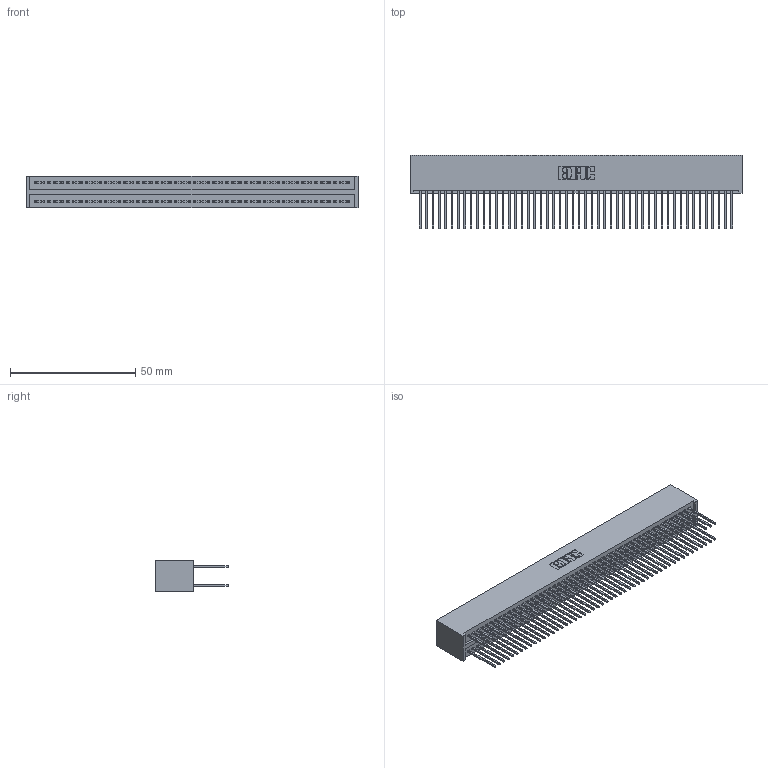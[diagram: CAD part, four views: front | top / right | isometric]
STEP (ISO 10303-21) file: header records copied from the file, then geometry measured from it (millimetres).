
FILE_DESCRIPTION (( 'STEP AP203' ), '1' );
FILE_NAME ('325-100-540-201.STEP', '2020-02-25T06:40:36', ( '' ), ( '' ), 'SwSTEP 2.0', 'SolidWorks 2016', '' );
FILE_SCHEMA (( 'CONFIG_CONTROL_DESIGN' ));
Length unit declared in the file: inch
Products named in the file (3): 325-100-540-201; 325-292-001_325-293-140; 325 Part_Lugless
Assembly tree (101 placements, depth 2):
  325-100-540-201
    325 Part_Lugless
    325-292-001_325-293-140  x100
Bounding box: 132.64 x 29.46 x 12.45 mm (x, y, z)
Volume: 18180.4 mm3; surface area: 24660.2 mm2
Topology: 101 solids, 101 shells, 5306 faces, 15787 edges, 10390 vertices
Faces by surface type: plane 3666, cylinder 1640
Entity records: 30873 total; most frequent: CARTESIAN_POINT 5106, ORIENTED_EDGE 5042, DIRECTION 4341, EDGE_CURVE 2521, LINE 2401, VECTOR 2401, VERTEX_POINT 1678, AXIS2_PLACEMENT_3D 970
